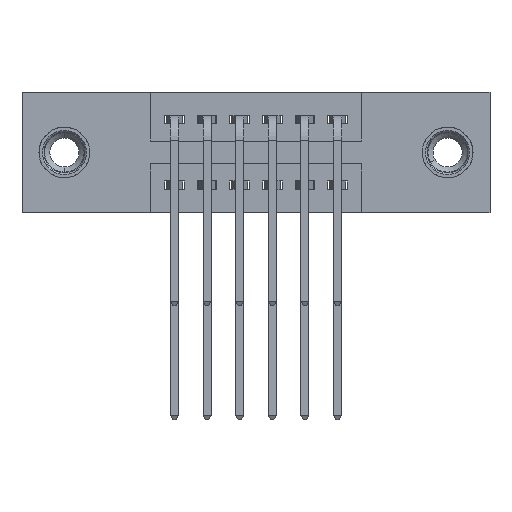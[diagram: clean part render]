
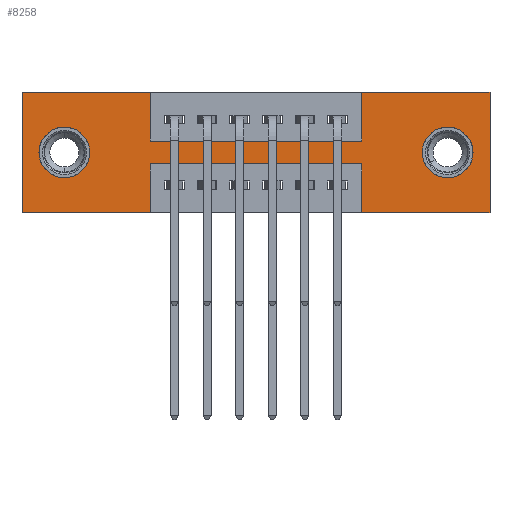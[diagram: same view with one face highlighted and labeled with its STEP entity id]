
A CAD part, front view. The second image highlights one B-rep face of the part: STEP entity #8258.
In plain terms, the highlighted planar face has unit normal (0, -1, 0).
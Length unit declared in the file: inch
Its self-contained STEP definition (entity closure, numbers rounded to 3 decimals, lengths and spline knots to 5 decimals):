
#30 = LINE ( 'NONE', #5247, #7189 ) ;
#140 = EDGE_CURVE ( 'NONE', #4086, #7706, #4077, .T. ) ;
#274 = DIRECTION ( 'NONE',  ( 0., 0., -1. ) ) ;
#293 = EDGE_LOOP ( 'NONE', ( #9547, #8868, #9456, #1589, #9748, #8150, #6167, #12147, #7324, #501, #10411, #7777 ) ) ;
#327 = DIRECTION ( 'NONE',  ( -1., 0., 0. ) ) ;
#501 = ORIENTED_EDGE ( 'NONE', *, *, #5644, .F. ) ;
#504 = CARTESIAN_POINT ( 'NONE',  ( 0., 0., -0.37 ) ) ;
#506 = EDGE_CURVE ( 'NONE', #7706, #4086, #2666, .T. ) ;
#671 = CARTESIAN_POINT ( 'NONE',  ( 1.0425, 0., -0.15 ) ) ;
#711 = DIRECTION ( 'NONE',  ( 1., 0., 0. ) ) ;
#1313 = LINE ( 'NONE', #11319, #6146 ) ;
#1334 = CARTESIAN_POINT ( 'NONE',  ( 1.0425, 0., -0.37 ) ) ;
#1342 = LINE ( 'NONE', #1736, #3651 ) ;
#1532 = EDGE_CURVE ( 'NONE', #5799, #5614, #12100, .T. ) ;
#1589 = ORIENTED_EDGE ( 'NONE', *, *, #2000, .F. ) ;
#1736 = CARTESIAN_POINT ( 'NONE',  ( 0., 0., 0. ) ) ;
#1773 = VERTEX_POINT ( 'NONE', #4814 ) ;
#1951 = FACE_OUTER_BOUND ( 'NONE', #293, .T. ) ;
#2000 = EDGE_CURVE ( 'NONE', #2122, #9489, #9290, .T. ) ;
#2118 = EDGE_CURVE ( 'NONE', #8813, #9513, #3409, .T. ) ;
#2122 = VERTEX_POINT ( 'NONE', #10097 ) ;
#2225 = LINE ( 'NONE', #6132, #5129 ) ;
#2640 = CARTESIAN_POINT ( 'NONE',  ( 1.435, 0., 0. ) ) ;
#2666 = CIRCLE ( 'NONE', #10106, 0.078 ) ;
#2675 = DIRECTION ( 'NONE',  ( 0., 0., 1. ) ) ;
#2785 = DIRECTION ( 'NONE',  ( -1., 0., 0. ) ) ;
#2878 = VERTEX_POINT ( 'NONE', #3382 ) ;
#2994 = CARTESIAN_POINT ( 'NONE',  ( 0., 0., 0. ) ) ;
#3044 = CIRCLE ( 'NONE', #3527, 0.078 ) ;
#3111 = CARTESIAN_POINT ( 'NONE',  ( 0., 0., 0. ) ) ;
#3327 = CARTESIAN_POINT ( 'NONE',  ( 1.435, 0., 0. ) ) ;
#3382 = CARTESIAN_POINT ( 'NONE',  ( 1.305, 0., -0.263 ) ) ;
#3394 = CARTESIAN_POINT ( 'NONE',  ( 0.3925, 0., -0.37 ) ) ;
#3409 = LINE ( 'NONE', #10190, #3716 ) ;
#3514 = VECTOR ( 'NONE', #3968, 39.37008 ) ;
#3527 = AXIS2_PLACEMENT_3D ( 'NONE', #3709, #10270, #4701 ) ;
#3624 = AXIS2_PLACEMENT_3D ( 'NONE', #4147, #10701, #5117 ) ;
#3651 = VECTOR ( 'NONE', #711, 39.37008 ) ;
#3683 = CARTESIAN_POINT ( 'NONE',  ( 0., 0., -0.37 ) ) ;
#3709 = CARTESIAN_POINT ( 'NONE',  ( 1.305, 0., -0.185 ) ) ;
#3716 = VECTOR ( 'NONE', #10123, 39.37008 ) ;
#3926 = EDGE_CURVE ( 'NONE', #9513, #6359, #9245, .T. ) ;
#3963 = CARTESIAN_POINT ( 'NONE',  ( 0.3925, 0., -0.15 ) ) ;
#3968 = DIRECTION ( 'NONE',  ( 0., 0., 1. ) ) ;
#3987 = EDGE_LOOP ( 'NONE', ( #4395, #8798 ) ) ;
#3997 = DIRECTION ( 'NONE',  ( 1., 0., 0. ) ) ;
#4077 = CIRCLE ( 'NONE', #7213, 0.078 ) ;
#4086 = VERTEX_POINT ( 'NONE', #6806 ) ;
#4147 = CARTESIAN_POINT ( 'NONE',  ( 1.305, 0., -0.185 ) ) ;
#4186 = VECTOR ( 'NONE', #10202, 39.37008 ) ;
#4395 = ORIENTED_EDGE ( 'NONE', *, *, #8558, .T. ) ;
#4671 = EDGE_CURVE ( 'NONE', #6359, #1773, #6790, .T. ) ;
#4701 = DIRECTION ( 'NONE',  ( 0., 0., -1. ) ) ;
#4814 = CARTESIAN_POINT ( 'NONE',  ( 0., 0., 0. ) ) ;
#5117 = DIRECTION ( 'NONE',  ( 0., 0., -1. ) ) ;
#5129 = VECTOR ( 'NONE', #274, 39.37008 ) ;
#5148 = CARTESIAN_POINT ( 'NONE',  ( 0.13, 0., -0.185 ) ) ;
#5247 = CARTESIAN_POINT ( 'NONE',  ( 0.3925, 0., -0.22 ) ) ;
#5268 = DIRECTION ( 'NONE',  ( 0., 0., 1. ) ) ;
#5295 = DIRECTION ( 'NONE',  ( 0., 1., 0. ) ) ;
#5614 = VERTEX_POINT ( 'NONE', #671 ) ;
#5620 = DIRECTION ( 'NONE',  ( 0., -1., 0. ) ) ;
#5644 = EDGE_CURVE ( 'NONE', #1773, #6614, #1342, .T. ) ;
#5739 = CARTESIAN_POINT ( 'NONE',  ( 0.3925, 0., 0. ) ) ;
#5799 = VERTEX_POINT ( 'NONE', #3963 ) ;
#5947 = ORIENTED_EDGE ( 'NONE', *, *, #140, .T. ) ;
#6018 = DIRECTION ( 'NONE',  ( 0., 0., 1. ) ) ;
#6047 = LINE ( 'NONE', #10519, #3514 ) ;
#6132 = CARTESIAN_POINT ( 'NONE',  ( 0.3925, 0., 0. ) ) ;
#6146 = VECTOR ( 'NONE', #12269, 39.37008 ) ;
#6167 = ORIENTED_EDGE ( 'NONE', *, *, #7260, .F. ) ;
#6310 = CIRCLE ( 'NONE', #3624, 0.078 ) ;
#6359 = VERTEX_POINT ( 'NONE', #504 ) ;
#6398 = AXIS2_PLACEMENT_3D ( 'NONE', #3683, #5620, #12140 ) ;
#6614 = VERTEX_POINT ( 'NONE', #5739 ) ;
#6751 = CARTESIAN_POINT ( 'NONE',  ( 1.0425, 0., -0.22 ) ) ;
#6790 = LINE ( 'NONE', #3111, #11445 ) ;
#6806 = CARTESIAN_POINT ( 'NONE',  ( 0.13, 0., -0.263 ) ) ;
#6829 = VECTOR ( 'NONE', #12033, 39.37008 ) ;
#7047 = FACE_BOUND ( 'NONE', #3987, .T. ) ;
#7107 = EDGE_CURVE ( 'NONE', #2878, #11762, #3044, .T. ) ;
#7189 = VECTOR ( 'NONE', #327, 39.37008 ) ;
#7213 = AXIS2_PLACEMENT_3D ( 'NONE', #12379, #12422, #2675 ) ;
#7260 = EDGE_CURVE ( 'NONE', #5614, #7599, #6047, .T. ) ;
#7324 = ORIENTED_EDGE ( 'NONE', *, *, #11848, .F. ) ;
#7435 = PLANE ( 'NONE',  #6398 ) ;
#7520 = CARTESIAN_POINT ( 'NONE',  ( 0., 0., -0.37 ) ) ;
#7599 = VERTEX_POINT ( 'NONE', #11939 ) ;
#7706 = VERTEX_POINT ( 'NONE', #8333 ) ;
#7777 = ORIENTED_EDGE ( 'NONE', *, *, #3926, .F. ) ;
#8021 = EDGE_CURVE ( 'NONE', #10456, #8813, #30, .T. ) ;
#8150 = ORIENTED_EDGE ( 'NONE', *, *, #11147, .F. ) ;
#8258 = ADVANCED_FACE ( 'NONE', ( #7047, #9216, #1951 ), #7435, .T. ) ;
#8333 = CARTESIAN_POINT ( 'NONE',  ( 0.13, 0., -0.107 ) ) ;
#8558 = EDGE_CURVE ( 'NONE', #11762, #2878, #6310, .T. ) ;
#8717 = VERTEX_POINT ( 'NONE', #3327 ) ;
#8731 = CARTESIAN_POINT ( 'NONE',  ( 1.305, 0., -0.107 ) ) ;
#8798 = ORIENTED_EDGE ( 'NONE', *, *, #7107, .T. ) ;
#8813 = VERTEX_POINT ( 'NONE', #10072 ) ;
#8826 = EDGE_LOOP ( 'NONE', ( #10867, #5947 ) ) ;
#8867 = VECTOR ( 'NONE', #3997, 39.37008 ) ;
#8868 = ORIENTED_EDGE ( 'NONE', *, *, #8021, .F. ) ;
#9216 = FACE_BOUND ( 'NONE', #8826, .T. ) ;
#9245 = LINE ( 'NONE', #7520, #11732 ) ;
#9290 = LINE ( 'NONE', #12092, #6829 ) ;
#9456 = ORIENTED_EDGE ( 'NONE', *, *, #9828, .F. ) ;
#9489 = VERTEX_POINT ( 'NONE', #1334 ) ;
#9513 = VERTEX_POINT ( 'NONE', #3394 ) ;
#9547 = ORIENTED_EDGE ( 'NONE', *, *, #2118, .F. ) ;
#9588 = VECTOR ( 'NONE', #11281, 39.37008 ) ;
#9748 = ORIENTED_EDGE ( 'NONE', *, *, #11560, .F. ) ;
#9828 = EDGE_CURVE ( 'NONE', #9489, #10456, #1313, .T. ) ;
#10072 = CARTESIAN_POINT ( 'NONE',  ( 0.3925, 0., -0.22 ) ) ;
#10097 = CARTESIAN_POINT ( 'NONE',  ( 1.435, 0., -0.37 ) ) ;
#10106 = AXIS2_PLACEMENT_3D ( 'NONE', #5148, #5295, #5268 ) ;
#10123 = DIRECTION ( 'NONE',  ( 0., 0., -1. ) ) ;
#10190 = CARTESIAN_POINT ( 'NONE',  ( 0.3925, 0., -0.37 ) ) ;
#10202 = DIRECTION ( 'NONE',  ( 0., 0., -1. ) ) ;
#10270 = DIRECTION ( 'NONE',  ( 0., 1., 0. ) ) ;
#10411 = ORIENTED_EDGE ( 'NONE', *, *, #4671, .F. ) ;
#10456 = VERTEX_POINT ( 'NONE', #6751 ) ;
#10519 = CARTESIAN_POINT ( 'NONE',  ( 1.0425, 0., 0. ) ) ;
#10701 = DIRECTION ( 'NONE',  ( 0., 1., 0. ) ) ;
#10812 = CARTESIAN_POINT ( 'NONE',  ( 0.3925, 0., -0.15 ) ) ;
#10867 = ORIENTED_EDGE ( 'NONE', *, *, #506, .T. ) ;
#11147 = EDGE_CURVE ( 'NONE', #7599, #8717, #11366, .T. ) ;
#11281 = DIRECTION ( 'NONE',  ( 1., 0., 0. ) ) ;
#11319 = CARTESIAN_POINT ( 'NONE',  ( 1.0425, 0., -0.37 ) ) ;
#11366 = LINE ( 'NONE', #2994, #8867 ) ;
#11445 = VECTOR ( 'NONE', #6018, 39.37008 ) ;
#11560 = EDGE_CURVE ( 'NONE', #8717, #2122, #11635, .T. ) ;
#11635 = LINE ( 'NONE', #2640, #4186 ) ;
#11732 = VECTOR ( 'NONE', #2785, 39.37008 ) ;
#11762 = VERTEX_POINT ( 'NONE', #8731 ) ;
#11848 = EDGE_CURVE ( 'NONE', #6614, #5799, #2225, .T. ) ;
#11939 = CARTESIAN_POINT ( 'NONE',  ( 1.0425, 0., 0. ) ) ;
#12033 = DIRECTION ( 'NONE',  ( -1., 0., 0. ) ) ;
#12092 = CARTESIAN_POINT ( 'NONE',  ( 0., 0., -0.37 ) ) ;
#12100 = LINE ( 'NONE', #10812, #9588 ) ;
#12140 = DIRECTION ( 'NONE',  ( 0., 0., -1. ) ) ;
#12147 = ORIENTED_EDGE ( 'NONE', *, *, #1532, .F. ) ;
#12269 = DIRECTION ( 'NONE',  ( 0., 0., 1. ) ) ;
#12379 = CARTESIAN_POINT ( 'NONE',  ( 0.13, 0., -0.185 ) ) ;
#12422 = DIRECTION ( 'NONE',  ( 0., 1., 0. ) ) ;
